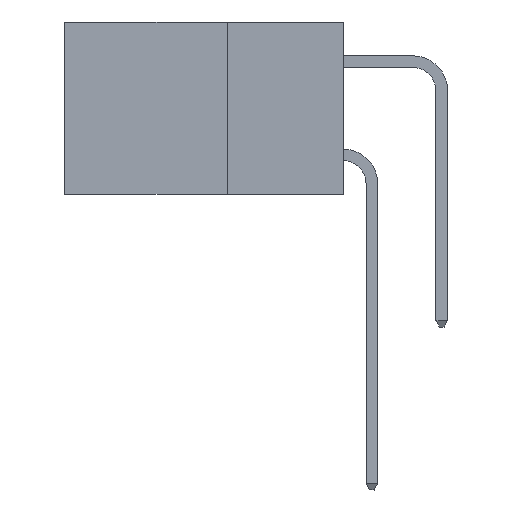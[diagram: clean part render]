
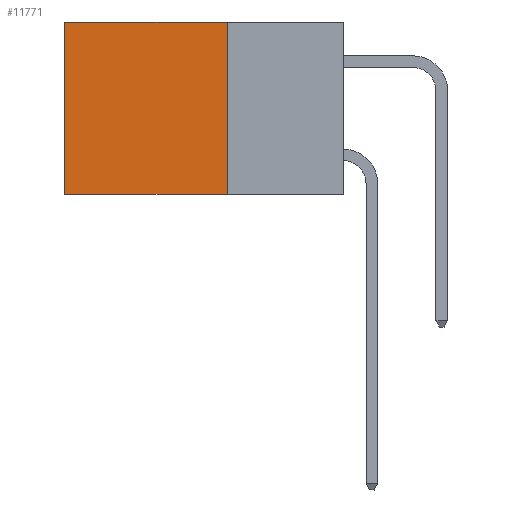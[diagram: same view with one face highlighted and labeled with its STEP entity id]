
A CAD part, left-side view. The second image highlights one B-rep face of the part: STEP entity #11771.
In plain terms, the highlighted planar face has unit normal (-1, 0, 0).
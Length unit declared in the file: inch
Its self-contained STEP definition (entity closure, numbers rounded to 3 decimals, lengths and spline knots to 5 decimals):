
#3187 = DIRECTION ( 'NONE',  ( 0., 0., -1. ) ) ;
#3400 = AXIS2_PLACEMENT_3D ( 'NONE', #4623, #32988, #30095 ) ;
#4250 = EDGE_CURVE ( 'NONE', #28284, #15140, #22155, .T. ) ;
#4553 = CARTESIAN_POINT ( 'NONE',  ( 0.298, 0.25, 0. ) ) ;
#4623 = CARTESIAN_POINT ( 'NONE',  ( 0.298, 0.25, 0. ) ) ;
#5618 = VECTOR ( 'NONE', #3187, 39.37008 ) ;
#8467 = EDGE_CURVE ( 'NONE', #16990, #26975, #29655, .T. ) ;
#9403 = DIRECTION ( 'NONE',  ( 0., 0., -1. ) ) ;
#10217 = VECTOR ( 'NONE', #17014, 39.37008 ) ;
#10218 = CARTESIAN_POINT ( 'NONE',  ( 0.298, 0.25, 0. ) ) ;
#11744 = VECTOR ( 'NONE', #9403, 39.37008 ) ;
#11771 = ADVANCED_FACE ( 'NONE', ( #29328 ), #32662, .F. ) ;
#12381 = LINE ( 'NONE', #18552, #5618 ) ;
#12524 = CARTESIAN_POINT ( 'NONE',  ( 0.298, 0.25, -0.37 ) ) ;
#12930 = LINE ( 'NONE', #17190, #11744 ) ;
#15140 = VERTEX_POINT ( 'NONE', #26444 ) ;
#15395 = ORIENTED_EDGE ( 'NONE', *, *, #32923, .F. ) ;
#16990 = VERTEX_POINT ( 'NONE', #21168 ) ;
#17014 = DIRECTION ( 'NONE',  ( 0., 1., 0. ) ) ;
#17190 = CARTESIAN_POINT ( 'NONE',  ( 0.298, 0.6, 0. ) ) ;
#17197 = VECTOR ( 'NONE', #20305, 39.37008 ) ;
#18552 = CARTESIAN_POINT ( 'NONE',  ( 0.298, 0.25, 0. ) ) ;
#19959 = CARTESIAN_POINT ( 'NONE',  ( 0.298, 0.6, -0.37 ) ) ;
#20305 = DIRECTION ( 'NONE',  ( 0., 1., 0. ) ) ;
#20465 = ORIENTED_EDGE ( 'NONE', *, *, #8467, .F. ) ;
#21168 = CARTESIAN_POINT ( 'NONE',  ( 0.298, 0.25, -0.37 ) ) ;
#21384 = EDGE_CURVE ( 'NONE', #15140, #26975, #12930, .T. ) ;
#22155 = LINE ( 'NONE', #4553, #10217 ) ;
#22515 = ORIENTED_EDGE ( 'NONE', *, *, #21384, .T. ) ;
#26305 = EDGE_LOOP ( 'NONE', ( #22515, #20465, #15395, #29214 ) ) ;
#26444 = CARTESIAN_POINT ( 'NONE',  ( 0.298, 0.6, 0. ) ) ;
#26975 = VERTEX_POINT ( 'NONE', #19959 ) ;
#28284 = VERTEX_POINT ( 'NONE', #10218 ) ;
#29214 = ORIENTED_EDGE ( 'NONE', *, *, #4250, .T. ) ;
#29328 = FACE_OUTER_BOUND ( 'NONE', #26305, .T. ) ;
#29655 = LINE ( 'NONE', #12524, #17197 ) ;
#30095 = DIRECTION ( 'NONE',  ( 0., 0., -1. ) ) ;
#32662 = PLANE ( 'NONE',  #3400 ) ;
#32923 = EDGE_CURVE ( 'NONE', #28284, #16990, #12381, .T. ) ;
#32988 = DIRECTION ( 'NONE',  ( 1., 0., 0. ) ) ;
